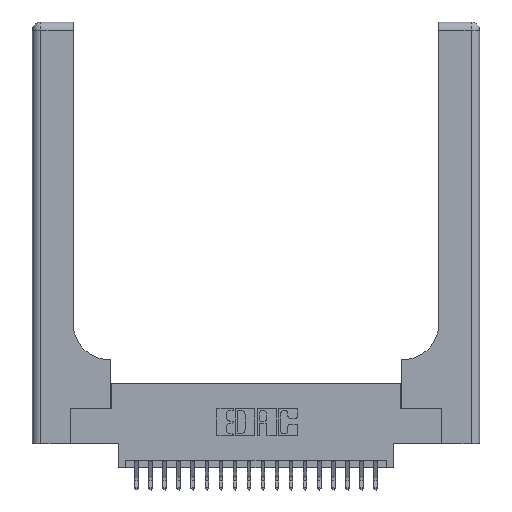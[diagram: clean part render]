
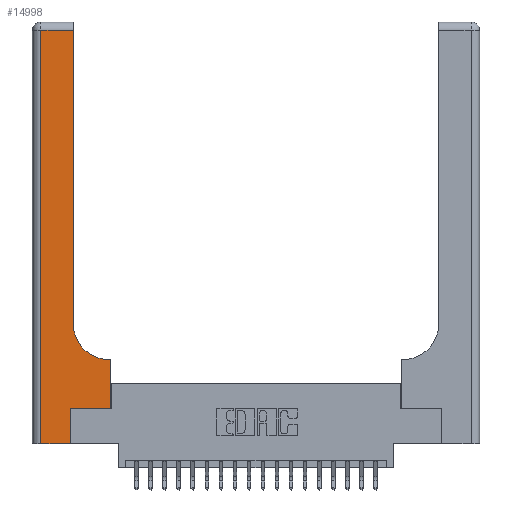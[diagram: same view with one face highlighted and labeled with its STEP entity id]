
A CAD part, top view. The second image highlights one B-rep face of the part: STEP entity #14998.
In plain terms, the highlighted planar face has unit normal (0, 0, 1).
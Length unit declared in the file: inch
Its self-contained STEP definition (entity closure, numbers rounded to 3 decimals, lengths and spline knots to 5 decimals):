
#182 = CARTESIAN_POINT ( 'NONE',  ( 0.5585, 0.25, 0.37 ) ) ;
#533 = CARTESIAN_POINT ( 'NONE',  ( 0.269, 0., 0.37 ) ) ;
#1086 = EDGE_LOOP ( 'NONE', ( #1935, #17398, #14682, #7974, #20841, #2257, #5020, #19614, #11639 ) ) ;
#1107 = VERTEX_POINT ( 'NONE', #7537 ) ;
#1280 = DIRECTION ( 'NONE',  ( 1., 0., 0. ) ) ;
#1333 = CARTESIAN_POINT ( 'NONE',  ( 0., 0., 0.37 ) ) ;
#1606 = PLANE ( 'NONE',  #18568 ) ;
#1874 = CARTESIAN_POINT ( 'NONE',  ( 0.269, 0.25, 0.37 ) ) ;
#1935 = ORIENTED_EDGE ( 'NONE', *, *, #2282, .T. ) ;
#2257 = ORIENTED_EDGE ( 'NONE', *, *, #11623, .T. ) ;
#2282 = EDGE_CURVE ( 'NONE', #12434, #13684, #12275, .T. ) ;
#2418 = EDGE_CURVE ( 'NONE', #8837, #6193, #10044, .T. ) ;
#2421 = DIRECTION ( 'NONE',  ( 0., 1., 0. ) ) ;
#2470 = VERTEX_POINT ( 'NONE', #19037 ) ;
#2692 = VECTOR ( 'NONE', #7485, 39.37008 ) ;
#2864 = CIRCLE ( 'NONE', #3371, 0.25 ) ;
#3328 = LINE ( 'NONE', #15796, #3916 ) ;
#3371 = AXIS2_PLACEMENT_3D ( 'NONE', #7072, #19451, #8897 ) ;
#3427 = VECTOR ( 'NONE', #8489, 39.37008 ) ;
#3448 = CARTESIAN_POINT ( 'NONE',  ( 0., 3., 0.37 ) ) ;
#3880 = EDGE_CURVE ( 'NONE', #1107, #12434, #2864, .T. ) ;
#3916 = VECTOR ( 'NONE', #12182, 39.37008 ) ;
#4934 = CARTESIAN_POINT ( 'NONE',  ( 0., 2.94, 0.37 ) ) ;
#5020 = ORIENTED_EDGE ( 'NONE', *, *, #15179, .T. ) ;
#5066 = VECTOR ( 'NONE', #9984, 39.37008 ) ;
#5102 = VERTEX_POINT ( 'NONE', #8777 ) ;
#5241 = VECTOR ( 'NONE', #1280, 39.37008 ) ;
#5307 = DIRECTION ( 'NONE',  ( 0., 0., -1. ) ) ;
#6193 = VERTEX_POINT ( 'NONE', #10307 ) ;
#7013 = EDGE_CURVE ( 'NONE', #5102, #1107, #19228, .T. ) ;
#7072 = CARTESIAN_POINT ( 'NONE',  ( 0.5415, 0.85, 0.37 ) ) ;
#7485 = DIRECTION ( 'NONE',  ( 0., 1., 0. ) ) ;
#7537 = CARTESIAN_POINT ( 'NONE',  ( 0.5415, 0.6, 0.37 ) ) ;
#7974 = ORIENTED_EDGE ( 'NONE', *, *, #2418, .T. ) ;
#7985 = FACE_OUTER_BOUND ( 'NONE', #1086, .T. ) ;
#8032 = VECTOR ( 'NONE', #8184, 39.37008 ) ;
#8184 = DIRECTION ( 'NONE',  ( 0., 1., 0. ) ) ;
#8252 = LINE ( 'NONE', #20746, #3427 ) ;
#8489 = DIRECTION ( 'NONE',  ( 0., -1., 0. ) ) ;
#8777 = CARTESIAN_POINT ( 'NONE',  ( 0.5585, 0.6, 0.37 ) ) ;
#8837 = VERTEX_POINT ( 'NONE', #15072 ) ;
#8897 = DIRECTION ( 'NONE',  ( 1., 0., 0. ) ) ;
#9133 = VERTEX_POINT ( 'NONE', #19556 ) ;
#9720 = VECTOR ( 'NONE', #19132, 39.37008 ) ;
#9984 = DIRECTION ( 'NONE',  ( -1., 0., 0. ) ) ;
#10044 = LINE ( 'NONE', #1333, #5241 ) ;
#10161 = EDGE_CURVE ( 'NONE', #6193, #11828, #17975, .T. ) ;
#10307 = CARTESIAN_POINT ( 'NONE',  ( 0.269, 0., 0.37 ) ) ;
#10766 = CARTESIAN_POINT ( 'NONE',  ( 0.2915, 0.85, 0.37 ) ) ;
#11623 = EDGE_CURVE ( 'NONE', #11828, #9133, #3328, .T. ) ;
#11639 = ORIENTED_EDGE ( 'NONE', *, *, #3880, .T. ) ;
#11828 = VERTEX_POINT ( 'NONE', #1874 ) ;
#12182 = DIRECTION ( 'NONE',  ( 1., 0., 0. ) ) ;
#12275 = LINE ( 'NONE', #12425, #8032 ) ;
#12425 = CARTESIAN_POINT ( 'NONE',  ( 0.2915, 3., 0.37 ) ) ;
#12434 = VERTEX_POINT ( 'NONE', #10766 ) ;
#13253 = VECTOR ( 'NONE', #2421, 39.37008 ) ;
#13684 = VERTEX_POINT ( 'NONE', #14323 ) ;
#14323 = CARTESIAN_POINT ( 'NONE',  ( 0.2915, 2.94, 0.37 ) ) ;
#14481 = LINE ( 'NONE', #4934, #9720 ) ;
#14682 = ORIENTED_EDGE ( 'NONE', *, *, #18549, .T. ) ;
#14872 = EDGE_CURVE ( 'NONE', #13684, #2470, #14481, .T. ) ;
#14998 = ADVANCED_FACE ( 'NONE', ( #7985 ), #1606, .F. ) ;
#15072 = CARTESIAN_POINT ( 'NONE',  ( 0.06, 0., 0.37 ) ) ;
#15179 = EDGE_CURVE ( 'NONE', #9133, #5102, #21471, .T. ) ;
#15796 = CARTESIAN_POINT ( 'NONE',  ( 0.269, 0.25, 0.37 ) ) ;
#17398 = ORIENTED_EDGE ( 'NONE', *, *, #14872, .T. ) ;
#17835 = DIRECTION ( 'NONE',  ( -1., 0., 0. ) ) ;
#17975 = LINE ( 'NONE', #533, #13253 ) ;
#18549 = EDGE_CURVE ( 'NONE', #2470, #8837, #8252, .T. ) ;
#18568 = AXIS2_PLACEMENT_3D ( 'NONE', #3448, #5307, #17835 ) ;
#18788 = CARTESIAN_POINT ( 'NONE',  ( 0.2915, 0.6, 0.37 ) ) ;
#19037 = CARTESIAN_POINT ( 'NONE',  ( 0.06, 2.94, 0.37 ) ) ;
#19132 = DIRECTION ( 'NONE',  ( -1., 0., 0. ) ) ;
#19228 = LINE ( 'NONE', #18788, #5066 ) ;
#19451 = DIRECTION ( 'NONE',  ( 0., 0., -1. ) ) ;
#19556 = CARTESIAN_POINT ( 'NONE',  ( 0.5585, 0.25, 0.37 ) ) ;
#19614 = ORIENTED_EDGE ( 'NONE', *, *, #7013, .T. ) ;
#20746 = CARTESIAN_POINT ( 'NONE',  ( 0.06, 3., 0.37 ) ) ;
#20841 = ORIENTED_EDGE ( 'NONE', *, *, #10161, .T. ) ;
#21471 = LINE ( 'NONE', #182, #2692 ) ;
